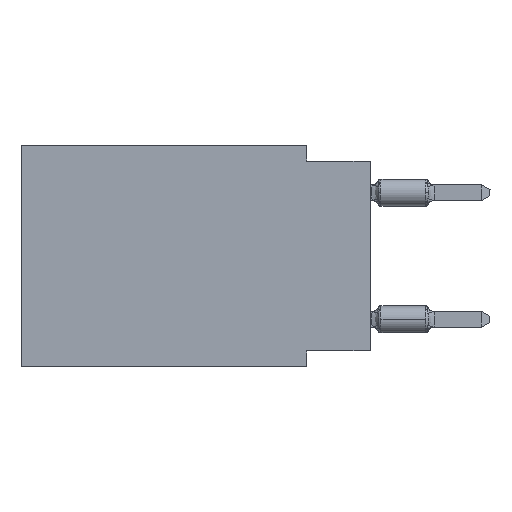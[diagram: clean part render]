
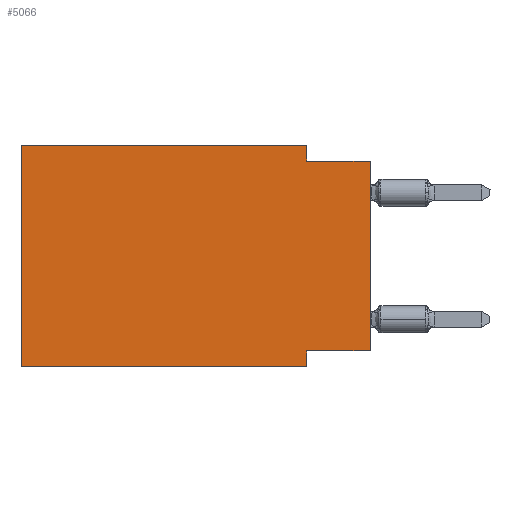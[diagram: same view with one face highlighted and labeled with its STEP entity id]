
A CAD part, left-side view. The second image highlights one B-rep face of the part: STEP entity #5066.
In plain terms, the highlighted planar face has unit normal (-1, 0, 0).
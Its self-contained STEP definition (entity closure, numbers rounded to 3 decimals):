
#265 = LINE ( 'NONE', #14338, #25964 ) ;
#275 = CARTESIAN_POINT ( 'NONE',  ( 0., 13.97, 0. ) ) ;
#637 = DIRECTION ( 'NONE',  ( 0., 1., 0. ) ) ;
#2028 = DIRECTION ( 'NONE',  ( 0., 0., -1. ) ) ;
#2166 = ORIENTED_EDGE ( 'NONE', *, *, #21231, .F. ) ;
#2497 = CARTESIAN_POINT ( 'NONE',  ( 0., 0., -8.255 ) ) ;
#3048 = ORIENTED_EDGE ( 'NONE', *, *, #25770, .F. ) ;
#3429 = LINE ( 'NONE', #11521, #21357 ) ;
#3546 = VECTOR ( 'NONE', #13998, 1000. ) ;
#3896 = CARTESIAN_POINT ( 'NONE',  ( 0., 2.54, -0.635 ) ) ;
#4384 = DIRECTION ( 'NONE',  ( 1., 0., 0. ) ) ;
#4646 = VERTEX_POINT ( 'NONE', #16878 ) ;
#4928 = LINE ( 'NONE', #21099, #12477 ) ;
#5066 = ADVANCED_FACE ( 'NONE', ( #24678 ), #20809, .F. ) ;
#6423 = VERTEX_POINT ( 'NONE', #19360 ) ;
#6718 = CARTESIAN_POINT ( 'NONE',  ( 0., 13.97, 0. ) ) ;
#7901 = CARTESIAN_POINT ( 'NONE',  ( 0., 0., 0. ) ) ;
#7920 = EDGE_CURVE ( 'NONE', #17600, #15290, #16564, .T. ) ;
#8371 = DIRECTION ( 'NONE',  ( 0., 0., -1. ) ) ;
#9424 = DIRECTION ( 'NONE',  ( 0., -1., 0. ) ) ;
#9551 = VERTEX_POINT ( 'NONE', #6718 ) ;
#9855 = VECTOR ( 'NONE', #2028, 1000. ) ;
#10075 = DIRECTION ( 'NONE',  ( 0., -1., 0. ) ) ;
#10124 = CARTESIAN_POINT ( 'NONE',  ( 0., 2.54, 0. ) ) ;
#10580 = EDGE_CURVE ( 'NONE', #4646, #12418, #4928, .T. ) ;
#11285 = ORIENTED_EDGE ( 'NONE', *, *, #22005, .F. ) ;
#11521 = CARTESIAN_POINT ( 'NONE',  ( 0., 0., -0.635 ) ) ;
#11575 = EDGE_LOOP ( 'NONE', ( #13949, #3048, #11285, #18612, #22877, #20150, #2166, #25809 ) ) ;
#11713 = VERTEX_POINT ( 'NONE', #13730 ) ;
#11893 = VERTEX_POINT ( 'NONE', #3896 ) ;
#12042 = LINE ( 'NONE', #24143, #13265 ) ;
#12195 = CARTESIAN_POINT ( 'NONE',  ( 0., 2.54, -8.255 ) ) ;
#12418 = VERTEX_POINT ( 'NONE', #14982 ) ;
#12477 = VECTOR ( 'NONE', #9424, 1000. ) ;
#13265 = VECTOR ( 'NONE', #10075, 1000. ) ;
#13730 = CARTESIAN_POINT ( 'NONE',  ( 0., 0., -0.635 ) ) ;
#13949 = ORIENTED_EDGE ( 'NONE', *, *, #23496, .T. ) ;
#13998 = DIRECTION ( 'NONE',  ( 0., 0., 1. ) ) ;
#14337 = DIRECTION ( 'NONE',  ( 0., 0., -1. ) ) ;
#14338 = CARTESIAN_POINT ( 'NONE',  ( 0., 13.97, 0. ) ) ;
#14982 = CARTESIAN_POINT ( 'NONE',  ( 0., 2.54, -8.89 ) ) ;
#15213 = EDGE_CURVE ( 'NONE', #9551, #6423, #12042, .T. ) ;
#15290 = VERTEX_POINT ( 'NONE', #12195 ) ;
#15380 = CARTESIAN_POINT ( 'NONE',  ( 0., 0., -8.255 ) ) ;
#16318 = LINE ( 'NONE', #24422, #21674 ) ;
#16455 = DIRECTION ( 'NONE',  ( 0., 0., 1. ) ) ;
#16564 = LINE ( 'NONE', #2497, #21974 ) ;
#16878 = CARTESIAN_POINT ( 'NONE',  ( 0., 13.97, -8.89 ) ) ;
#17490 = AXIS2_PLACEMENT_3D ( 'NONE', #275, #4384, #8371 ) ;
#17600 = VERTEX_POINT ( 'NONE', #15380 ) ;
#18612 = ORIENTED_EDGE ( 'NONE', *, *, #15213, .F. ) ;
#19360 = CARTESIAN_POINT ( 'NONE',  ( 0., 2.54, 0. ) ) ;
#19600 = DIRECTION ( 'NONE',  ( 0., -1., 0. ) ) ;
#20150 = ORIENTED_EDGE ( 'NONE', *, *, #10580, .T. ) ;
#20809 = PLANE ( 'NONE',  #17490 ) ;
#21099 = CARTESIAN_POINT ( 'NONE',  ( 0., 13.97, -8.89 ) ) ;
#21231 = EDGE_CURVE ( 'NONE', #15290, #12418, #16318, .T. ) ;
#21357 = VECTOR ( 'NONE', #19600, 1000. ) ;
#21674 = VECTOR ( 'NONE', #14337, 1000. ) ;
#21974 = VECTOR ( 'NONE', #637, 1000. ) ;
#22005 = EDGE_CURVE ( 'NONE', #6423, #11893, #22720, .T. ) ;
#22375 = EDGE_CURVE ( 'NONE', #4646, #9551, #265, .T. ) ;
#22720 = LINE ( 'NONE', #10124, #9855 ) ;
#22877 = ORIENTED_EDGE ( 'NONE', *, *, #22375, .F. ) ;
#23496 = EDGE_CURVE ( 'NONE', #17600, #11713, #24079, .T. ) ;
#24079 = LINE ( 'NONE', #7901, #3546 ) ;
#24143 = CARTESIAN_POINT ( 'NONE',  ( 0., 13.97, 0. ) ) ;
#24422 = CARTESIAN_POINT ( 'NONE',  ( 0., 2.54, -8.89 ) ) ;
#24678 = FACE_OUTER_BOUND ( 'NONE', #11575, .T. ) ;
#25770 = EDGE_CURVE ( 'NONE', #11893, #11713, #3429, .T. ) ;
#25809 = ORIENTED_EDGE ( 'NONE', *, *, #7920, .F. ) ;
#25964 = VECTOR ( 'NONE', #16455, 1000. ) ;
